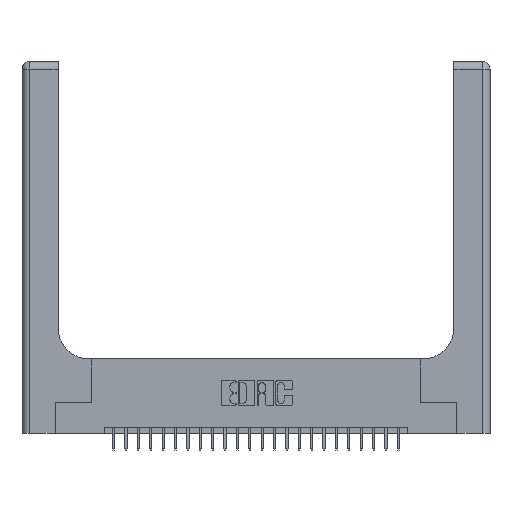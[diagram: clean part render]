
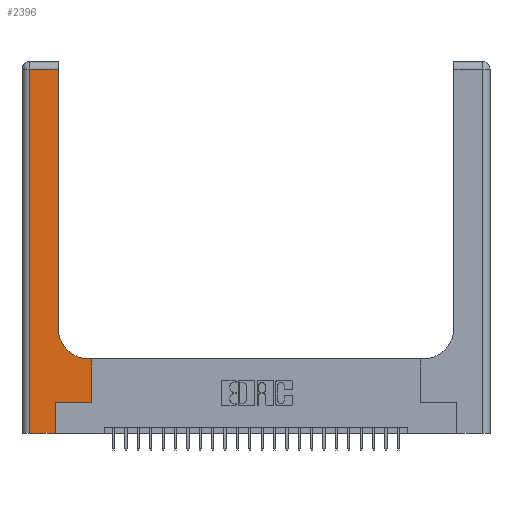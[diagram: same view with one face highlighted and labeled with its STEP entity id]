
A CAD part, top view. The second image highlights one B-rep face of the part: STEP entity #2396.
In plain terms, the highlighted planar face has unit normal (0, 0, 1).
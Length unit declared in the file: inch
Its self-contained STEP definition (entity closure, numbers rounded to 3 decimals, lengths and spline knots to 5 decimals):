
#90 = FACE_OUTER_BOUND ( 'NONE', #11701, .T. ) ;
#650 = CARTESIAN_POINT ( 'NONE',  ( 0., 0., 0.37 ) ) ;
#778 = CARTESIAN_POINT ( 'NONE',  ( 0., 2.94, 0.37 ) ) ;
#992 = CARTESIAN_POINT ( 'NONE',  ( 0.269, 0.25, 0.37 ) ) ;
#1036 = ORIENTED_EDGE ( 'NONE', *, *, #4661, .T. ) ;
#1087 = VERTEX_POINT ( 'NONE', #20184 ) ;
#1122 = DIRECTION ( 'NONE',  ( 1., 0., 0. ) ) ;
#2396 = ADVANCED_FACE ( 'NONE', ( #90 ), #7757, .F. ) ;
#2638 = CARTESIAN_POINT ( 'NONE',  ( 0.5415, 0.6, 0.37 ) ) ;
#2697 = DIRECTION ( 'NONE',  ( 0., 1., 0. ) ) ;
#2900 = CARTESIAN_POINT ( 'NONE',  ( 0.5415, 0.85, 0.37 ) ) ;
#4493 = ORIENTED_EDGE ( 'NONE', *, *, #6896, .T. ) ;
#4661 = EDGE_CURVE ( 'NONE', #23741, #20991, #24429, .T. ) ;
#4821 = ORIENTED_EDGE ( 'NONE', *, *, #16401, .T. ) ;
#5194 = DIRECTION ( 'NONE',  ( -1., 0., 0. ) ) ;
#5475 = ORIENTED_EDGE ( 'NONE', *, *, #7918, .T. ) ;
#5986 = ORIENTED_EDGE ( 'NONE', *, *, #9915, .T. ) ;
#6193 = CARTESIAN_POINT ( 'NONE',  ( 0.2915, 0.6, 0.37 ) ) ;
#6222 = ORIENTED_EDGE ( 'NONE', *, *, #7710, .T. ) ;
#6522 = EDGE_CURVE ( 'NONE', #15675, #16383, #15024, .T. ) ;
#6819 = CARTESIAN_POINT ( 'NONE',  ( 0.269, 0.25, 0.37 ) ) ;
#6896 = EDGE_CURVE ( 'NONE', #25817, #14027, #21152, .T. ) ;
#7053 = VECTOR ( 'NONE', #15037, 39.37008 ) ;
#7470 = CARTESIAN_POINT ( 'NONE',  ( 0.5585, 0.25, 0.37 ) ) ;
#7615 = CARTESIAN_POINT ( 'NONE',  ( 0.2915, 3., 0.37 ) ) ;
#7617 = AXIS2_PLACEMENT_3D ( 'NONE', #2900, #11105, #1122 ) ;
#7710 = EDGE_CURVE ( 'NONE', #1087, #25817, #8710, .T. ) ;
#7743 = ORIENTED_EDGE ( 'NONE', *, *, #18411, .T. ) ;
#7757 = PLANE ( 'NONE',  #14357 ) ;
#7918 = EDGE_CURVE ( 'NONE', #14981, #15675, #8028, .T. ) ;
#8028 = LINE ( 'NONE', #7615, #13554 ) ;
#8053 = VECTOR ( 'NONE', #11335, 39.37008 ) ;
#8169 = DIRECTION ( 'NONE',  ( 0., 0., -1. ) ) ;
#8298 = DIRECTION ( 'NONE',  ( -1., 0., 0. ) ) ;
#8503 = CIRCLE ( 'NONE', #7617, 0.25 ) ;
#8710 = LINE ( 'NONE', #650, #16533 ) ;
#9012 = CARTESIAN_POINT ( 'NONE',  ( 0.269, 0., 0.37 ) ) ;
#9914 = CARTESIAN_POINT ( 'NONE',  ( 0.269, 0., 0.37 ) ) ;
#9915 = EDGE_CURVE ( 'NONE', #25985, #14981, #8503, .T. ) ;
#10515 = VECTOR ( 'NONE', #2697, 39.37008 ) ;
#11105 = DIRECTION ( 'NONE',  ( 0., 0., -1. ) ) ;
#11335 = DIRECTION ( 'NONE',  ( 0., -1., 0. ) ) ;
#11359 = EDGE_CURVE ( 'NONE', #16383, #1087, #15217, .T. ) ;
#11428 = CARTESIAN_POINT ( 'NONE',  ( 0.06, 2.94, 0.37 ) ) ;
#11701 = EDGE_LOOP ( 'NONE', ( #5475, #14645, #14702, #6222, #4493, #4821, #1036, #7743, #5986 ) ) ;
#13554 = VECTOR ( 'NONE', #20420, 39.37008 ) ;
#13604 = CARTESIAN_POINT ( 'NONE',  ( 0.06, 3., 0.37 ) ) ;
#13938 = CARTESIAN_POINT ( 'NONE',  ( 0., 3., 0.37 ) ) ;
#14027 = VERTEX_POINT ( 'NONE', #992 ) ;
#14357 = AXIS2_PLACEMENT_3D ( 'NONE', #13938, #8169, #8298 ) ;
#14645 = ORIENTED_EDGE ( 'NONE', *, *, #6522, .T. ) ;
#14702 = ORIENTED_EDGE ( 'NONE', *, *, #11359, .T. ) ;
#14981 = VERTEX_POINT ( 'NONE', #15949 ) ;
#15024 = LINE ( 'NONE', #778, #22967 ) ;
#15037 = DIRECTION ( 'NONE',  ( 1., 0., 0. ) ) ;
#15217 = LINE ( 'NONE', #13604, #8053 ) ;
#15675 = VERTEX_POINT ( 'NONE', #26096 ) ;
#15949 = CARTESIAN_POINT ( 'NONE',  ( 0.2915, 0.85, 0.37 ) ) ;
#16036 = DIRECTION ( 'NONE',  ( -1., 0., 0. ) ) ;
#16383 = VERTEX_POINT ( 'NONE', #11428 ) ;
#16401 = EDGE_CURVE ( 'NONE', #14027, #23741, #25263, .T. ) ;
#16473 = VECTOR ( 'NONE', #16036, 39.37008 ) ;
#16533 = VECTOR ( 'NONE', #17049, 39.37008 ) ;
#17049 = DIRECTION ( 'NONE',  ( 1., 0., 0. ) ) ;
#18060 = LINE ( 'NONE', #6193, #16473 ) ;
#18411 = EDGE_CURVE ( 'NONE', #20991, #25985, #18060, .T. ) ;
#19209 = CARTESIAN_POINT ( 'NONE',  ( 0.5585, 0.6, 0.37 ) ) ;
#20021 = DIRECTION ( 'NONE',  ( 0., 1., 0. ) ) ;
#20184 = CARTESIAN_POINT ( 'NONE',  ( 0.06, 0., 0.37 ) ) ;
#20420 = DIRECTION ( 'NONE',  ( 0., 1., 0. ) ) ;
#20991 = VERTEX_POINT ( 'NONE', #19209 ) ;
#21152 = LINE ( 'NONE', #9012, #10515 ) ;
#22967 = VECTOR ( 'NONE', #5194, 39.37008 ) ;
#23292 = CARTESIAN_POINT ( 'NONE',  ( 0.5585, 0.25, 0.37 ) ) ;
#23741 = VERTEX_POINT ( 'NONE', #23292 ) ;
#24429 = LINE ( 'NONE', #7470, #25700 ) ;
#25263 = LINE ( 'NONE', #6819, #7053 ) ;
#25700 = VECTOR ( 'NONE', #20021, 39.37008 ) ;
#25817 = VERTEX_POINT ( 'NONE', #9914 ) ;
#25985 = VERTEX_POINT ( 'NONE', #2638 ) ;
#26096 = CARTESIAN_POINT ( 'NONE',  ( 0.2915, 2.94, 0.37 ) ) ;
